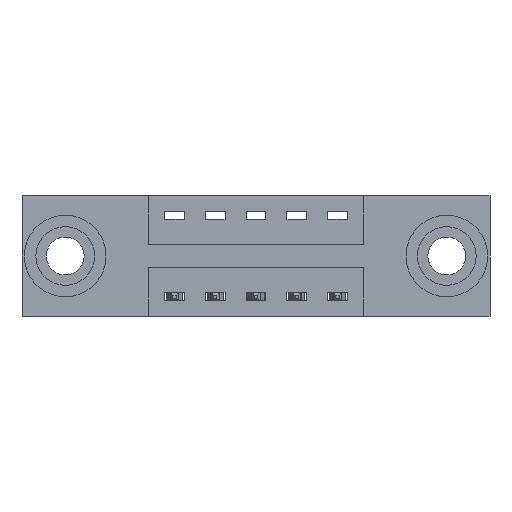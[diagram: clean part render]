
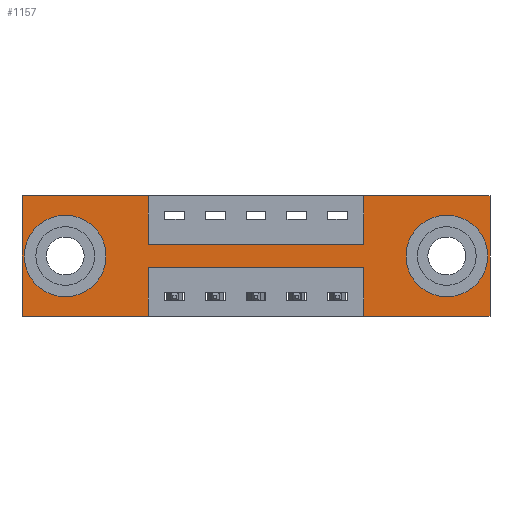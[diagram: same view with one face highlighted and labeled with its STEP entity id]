
A CAD part, front view. The second image highlights one B-rep face of the part: STEP entity #1157.
In plain terms, the highlighted planar face has unit normal (0, -1, 0).
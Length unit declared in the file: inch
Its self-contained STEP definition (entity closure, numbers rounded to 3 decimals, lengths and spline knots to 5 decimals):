
#103 = LINE ( 'NONE', #3554, #6271 ) ;
#162 = CIRCLE ( 'NONE', #2984, 0.078 ) ;
#208 = VERTEX_POINT ( 'NONE', #248 ) ;
#248 = CARTESIAN_POINT ( 'NONE',  ( 0.1325, 0., -0.107 ) ) ;
#315 = VERTEX_POINT ( 'NONE', #5360 ) ;
#372 = DIRECTION ( 'NONE',  ( 0., 0., -1. ) ) ;
#374 = CARTESIAN_POINT ( 'NONE',  ( 0., 0., -0.37 ) ) ;
#388 = VECTOR ( 'NONE', #2655, 39.37008 ) ;
#418 = FACE_BOUND ( 'NONE', #7819, .T. ) ;
#432 = CARTESIAN_POINT ( 'NONE',  ( 1.3025, 0., -0.185 ) ) ;
#462 = CIRCLE ( 'NONE', #8924, 0.078 ) ;
#463 = LINE ( 'NONE', #6097, #388 ) ;
#482 = DIRECTION ( 'NONE',  ( 0., 1., 0. ) ) ;
#567 = VECTOR ( 'NONE', #7456, 39.37008 ) ;
#683 = EDGE_CURVE ( 'NONE', #208, #315, #7086, .T. ) ;
#745 = CARTESIAN_POINT ( 'NONE',  ( 1.3025, 0., -0.107 ) ) ;
#951 = EDGE_CURVE ( 'NONE', #4273, #7753, #8706, .T. ) ;
#1157 = ADVANCED_FACE ( 'NONE', ( #8234, #418, #2508 ), #1908, .T. ) ;
#1176 = CARTESIAN_POINT ( 'NONE',  ( 1.0475, 0., -0.22 ) ) ;
#1255 = CARTESIAN_POINT ( 'NONE',  ( 0.3875, 0., -0.22 ) ) ;
#1304 = EDGE_CURVE ( 'NONE', #4823, #3530, #4171, .T. ) ;
#1408 = CARTESIAN_POINT ( 'NONE',  ( 0.3875, 0., -0.15 ) ) ;
#1495 = VECTOR ( 'NONE', #7578, 39.37008 ) ;
#1523 = EDGE_CURVE ( 'NONE', #4258, #7864, #8834, .T. ) ;
#1596 = EDGE_CURVE ( 'NONE', #3530, #4785, #7777, .T. ) ;
#1663 = ORIENTED_EDGE ( 'NONE', *, *, #7874, .F. ) ;
#1779 = EDGE_CURVE ( 'NONE', #7864, #4823, #2114, .T. ) ;
#1860 = LINE ( 'NONE', #7484, #2245 ) ;
#1863 = DIRECTION ( 'NONE',  ( 0., 0., -1. ) ) ;
#1865 = ORIENTED_EDGE ( 'NONE', *, *, #683, .T. ) ;
#1887 = ORIENTED_EDGE ( 'NONE', *, *, #2027, .F. ) ;
#1908 = PLANE ( 'NONE',  #7094 ) ;
#1998 = DIRECTION ( 'NONE',  ( 0., 0., -1. ) ) ;
#2027 = EDGE_CURVE ( 'NONE', #3049, #6136, #2219, .T. ) ;
#2052 = DIRECTION ( 'NONE',  ( -1., 0., 0. ) ) ;
#2114 = LINE ( 'NONE', #5419, #1495 ) ;
#2145 = EDGE_CURVE ( 'NONE', #4212, #3049, #1860, .T. ) ;
#2149 = ORIENTED_EDGE ( 'NONE', *, *, #1523, .F. ) ;
#2175 = DIRECTION ( 'NONE',  ( 1., 0., 0. ) ) ;
#2219 = LINE ( 'NONE', #2872, #6200 ) ;
#2245 = VECTOR ( 'NONE', #372, 39.37008 ) ;
#2275 = EDGE_CURVE ( 'NONE', #4785, #4273, #6511, .T. ) ;
#2340 = CARTESIAN_POINT ( 'NONE',  ( 0., 0., 0. ) ) ;
#2351 = EDGE_LOOP ( 'NONE', ( #6042, #3294, #7241, #2149, #8736, #4718, #1663, #1887, #6882, #6704, #7940, #5301 ) ) ;
#2368 = CARTESIAN_POINT ( 'NONE',  ( 0., 0., 0. ) ) ;
#2424 = EDGE_CURVE ( 'NONE', #4762, #4249, #6903, .T. ) ;
#2508 = FACE_OUTER_BOUND ( 'NONE', #2351, .T. ) ;
#2553 = VECTOR ( 'NONE', #3013, 39.37008 ) ;
#2655 = DIRECTION ( 'NONE',  ( 0., 0., 1. ) ) ;
#2677 = EDGE_LOOP ( 'NONE', ( #8053, #3616 ) ) ;
#2844 = DIRECTION ( 'NONE',  ( 1., 0., 0. ) ) ;
#2872 = CARTESIAN_POINT ( 'NONE',  ( 0.3875, 0., -0.15 ) ) ;
#2963 = AXIS2_PLACEMENT_3D ( 'NONE', #432, #6166, #1998 ) ;
#2984 = AXIS2_PLACEMENT_3D ( 'NONE', #5486, #482, #6873 ) ;
#3013 = DIRECTION ( 'NONE',  ( -1., 0., 0. ) ) ;
#3049 = VERTEX_POINT ( 'NONE', #1408 ) ;
#3218 = CARTESIAN_POINT ( 'NONE',  ( 0.3875, 0., 0. ) ) ;
#3294 = ORIENTED_EDGE ( 'NONE', *, *, #1304, .F. ) ;
#3508 = CARTESIAN_POINT ( 'NONE',  ( 0., 0., 0. ) ) ;
#3530 = VERTEX_POINT ( 'NONE', #4322 ) ;
#3554 = CARTESIAN_POINT ( 'NONE',  ( 0., 0., 0. ) ) ;
#3616 = ORIENTED_EDGE ( 'NONE', *, *, #5194, .T. ) ;
#3810 = CARTESIAN_POINT ( 'NONE',  ( 0., 0., -0.37 ) ) ;
#3852 = CIRCLE ( 'NONE', #2963, 0.078 ) ;
#3953 = CARTESIAN_POINT ( 'NONE',  ( 1.435, 0., 0. ) ) ;
#4085 = EDGE_CURVE ( 'NONE', #4862, #9043, #3852, .T. ) ;
#4171 = LINE ( 'NONE', #1255, #6636 ) ;
#4212 = VERTEX_POINT ( 'NONE', #3218 ) ;
#4249 = VERTEX_POINT ( 'NONE', #3953 ) ;
#4258 = VERTEX_POINT ( 'NONE', #6104 ) ;
#4273 = VERTEX_POINT ( 'NONE', #5471 ) ;
#4322 = CARTESIAN_POINT ( 'NONE',  ( 0.3875, 0., -0.22 ) ) ;
#4387 = DIRECTION ( 'NONE',  ( 1., 0., 0. ) ) ;
#4610 = VECTOR ( 'NONE', #2844, 39.37008 ) ;
#4674 = CARTESIAN_POINT ( 'NONE',  ( 1.0475, 0., -0.37 ) ) ;
#4718 = ORIENTED_EDGE ( 'NONE', *, *, #2424, .F. ) ;
#4739 = CARTESIAN_POINT ( 'NONE',  ( 0.3875, 0., -0.37 ) ) ;
#4762 = VERTEX_POINT ( 'NONE', #5833 ) ;
#4785 = VERTEX_POINT ( 'NONE', #8233 ) ;
#4823 = VERTEX_POINT ( 'NONE', #1176 ) ;
#4862 = VERTEX_POINT ( 'NONE', #745 ) ;
#5194 = EDGE_CURVE ( 'NONE', #9043, #4862, #162, .T. ) ;
#5209 = EDGE_CURVE ( 'NONE', #315, #208, #462, .T. ) ;
#5245 = DIRECTION ( 'NONE',  ( -1., 0., 0. ) ) ;
#5301 = ORIENTED_EDGE ( 'NONE', *, *, #2275, .F. ) ;
#5360 = CARTESIAN_POINT ( 'NONE',  ( 0.1325, 0., -0.263 ) ) ;
#5419 = CARTESIAN_POINT ( 'NONE',  ( 1.0475, 0., -0.37 ) ) ;
#5471 = CARTESIAN_POINT ( 'NONE',  ( 0., 0., -0.37 ) ) ;
#5486 = CARTESIAN_POINT ( 'NONE',  ( 1.3025, 0., -0.185 ) ) ;
#5608 = DIRECTION ( 'NONE',  ( 0., 0., -1. ) ) ;
#5678 = DIRECTION ( 'NONE',  ( 0., 1., 0. ) ) ;
#5833 = CARTESIAN_POINT ( 'NONE',  ( 1.0475, 0., 0. ) ) ;
#5974 = DIRECTION ( 'NONE',  ( 0., -1., 0. ) ) ;
#6042 = ORIENTED_EDGE ( 'NONE', *, *, #1596, .F. ) ;
#6097 = CARTESIAN_POINT ( 'NONE',  ( 1.0475, 0., 0. ) ) ;
#6104 = CARTESIAN_POINT ( 'NONE',  ( 1.435, 0., -0.37 ) ) ;
#6136 = VERTEX_POINT ( 'NONE', #6155 ) ;
#6155 = CARTESIAN_POINT ( 'NONE',  ( 1.0475, 0., -0.15 ) ) ;
#6158 = DIRECTION ( 'NONE',  ( 0., 0., -1. ) ) ;
#6164 = DIRECTION ( 'NONE',  ( 0., 1., 0. ) ) ;
#6166 = DIRECTION ( 'NONE',  ( 0., 1., 0. ) ) ;
#6200 = VECTOR ( 'NONE', #2175, 39.37008 ) ;
#6271 = VECTOR ( 'NONE', #4387, 39.37008 ) ;
#6434 = DIRECTION ( 'NONE',  ( 0., 0., 1. ) ) ;
#6511 = LINE ( 'NONE', #8719, #2553 ) ;
#6587 = EDGE_CURVE ( 'NONE', #4249, #4258, #7972, .T. ) ;
#6636 = VECTOR ( 'NONE', #2052, 39.37008 ) ;
#6664 = ORIENTED_EDGE ( 'NONE', *, *, #5209, .T. ) ;
#6704 = ORIENTED_EDGE ( 'NONE', *, *, #7335, .F. ) ;
#6873 = DIRECTION ( 'NONE',  ( 0., 0., -1. ) ) ;
#6882 = ORIENTED_EDGE ( 'NONE', *, *, #2145, .F. ) ;
#6903 = LINE ( 'NONE', #3508, #4610 ) ;
#6945 = VECTOR ( 'NONE', #6158, 39.37008 ) ;
#7086 = CIRCLE ( 'NONE', #9175, 0.078 ) ;
#7094 = AXIS2_PLACEMENT_3D ( 'NONE', #374, #5974, #1863 ) ;
#7096 = VECTOR ( 'NONE', #5245, 39.37008 ) ;
#7154 = CARTESIAN_POINT ( 'NONE',  ( 0.1325, 0., -0.185 ) ) ;
#7241 = ORIENTED_EDGE ( 'NONE', *, *, #1779, .F. ) ;
#7335 = EDGE_CURVE ( 'NONE', #7753, #4212, #103, .T. ) ;
#7455 = CARTESIAN_POINT ( 'NONE',  ( 1.3025, 0., -0.263 ) ) ;
#7456 = DIRECTION ( 'NONE',  ( 0., 0., 1. ) ) ;
#7484 = CARTESIAN_POINT ( 'NONE',  ( 0.3875, 0., 0. ) ) ;
#7578 = DIRECTION ( 'NONE',  ( 0., 0., 1. ) ) ;
#7753 = VERTEX_POINT ( 'NONE', #2340 ) ;
#7777 = LINE ( 'NONE', #4739, #6945 ) ;
#7819 = EDGE_LOOP ( 'NONE', ( #1865, #6664 ) ) ;
#7864 = VERTEX_POINT ( 'NONE', #4674 ) ;
#7874 = EDGE_CURVE ( 'NONE', #6136, #4762, #463, .T. ) ;
#7885 = CARTESIAN_POINT ( 'NONE',  ( 1.435, 0., 0. ) ) ;
#7940 = ORIENTED_EDGE ( 'NONE', *, *, #951, .F. ) ;
#7972 = LINE ( 'NONE', #7885, #8550 ) ;
#8053 = ORIENTED_EDGE ( 'NONE', *, *, #4085, .T. ) ;
#8233 = CARTESIAN_POINT ( 'NONE',  ( 0.3875, 0., -0.37 ) ) ;
#8234 = FACE_BOUND ( 'NONE', #2677, .T. ) ;
#8241 = CARTESIAN_POINT ( 'NONE',  ( 0.1325, 0., -0.185 ) ) ;
#8550 = VECTOR ( 'NONE', #5608, 39.37008 ) ;
#8706 = LINE ( 'NONE', #2368, #567 ) ;
#8719 = CARTESIAN_POINT ( 'NONE',  ( 0., 0., -0.37 ) ) ;
#8736 = ORIENTED_EDGE ( 'NONE', *, *, #6587, .F. ) ;
#8834 = LINE ( 'NONE', #3810, #7096 ) ;
#8924 = AXIS2_PLACEMENT_3D ( 'NONE', #8241, #6164, #9029 ) ;
#9029 = DIRECTION ( 'NONE',  ( 0., 0., 1. ) ) ;
#9043 = VERTEX_POINT ( 'NONE', #7455 ) ;
#9175 = AXIS2_PLACEMENT_3D ( 'NONE', #7154, #5678, #6434 ) ;
